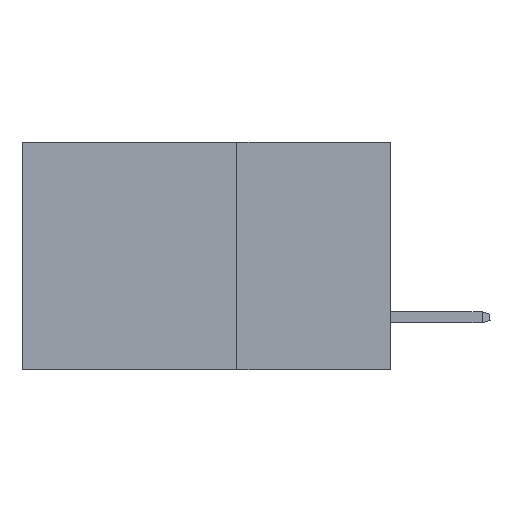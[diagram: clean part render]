
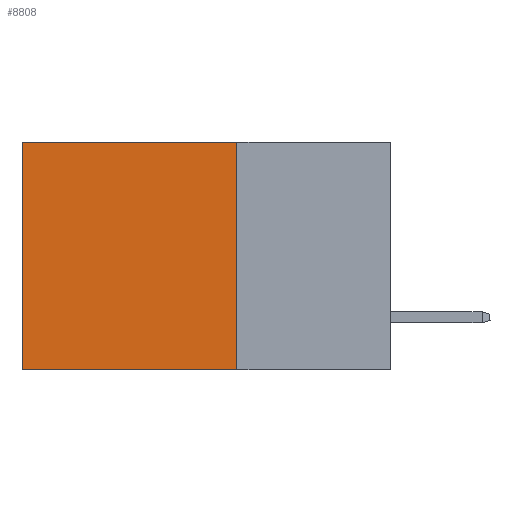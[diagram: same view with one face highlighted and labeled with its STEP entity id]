
A CAD part, left-side view. The second image highlights one B-rep face of the part: STEP entity #8808.
In plain terms, the highlighted planar face has unit normal (-1, 0, 0).
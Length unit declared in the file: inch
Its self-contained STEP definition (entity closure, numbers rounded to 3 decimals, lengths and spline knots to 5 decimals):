
#234 = EDGE_CURVE ( 'NONE', #16937, #2822, #19869, .T. ) ;
#302 = CARTESIAN_POINT ( 'NONE',  ( 0.2875, 0.6, 0. ) ) ;
#728 = CARTESIAN_POINT ( 'NONE',  ( 0.2875, 0.25, -0.37 ) ) ;
#2822 = VERTEX_POINT ( 'NONE', #15626 ) ;
#3097 = DIRECTION ( 'NONE',  ( 0., 0., -1. ) ) ;
#3258 = DIRECTION ( 'NONE',  ( 0., 0., -1. ) ) ;
#3316 = FACE_OUTER_BOUND ( 'NONE', #6712, .T. ) ;
#3740 = EDGE_CURVE ( 'NONE', #21979, #6977, #15382, .T. ) ;
#4184 = CARTESIAN_POINT ( 'NONE',  ( 0.2875, 0.25, 0. ) ) ;
#5078 = CARTESIAN_POINT ( 'NONE',  ( 0.2875, 0.6, 0. ) ) ;
#5442 = DIRECTION ( 'NONE',  ( 1., 0., 0. ) ) ;
#6490 = VECTOR ( 'NONE', #15784, 39.37008 ) ;
#6712 = EDGE_LOOP ( 'NONE', ( #21986, #18665, #23042, #12474 ) ) ;
#6977 = VERTEX_POINT ( 'NONE', #14801 ) ;
#8643 = LINE ( 'NONE', #728, #14646 ) ;
#8808 = ADVANCED_FACE ( 'NONE', ( #3316 ), #20551, .F. ) ;
#11276 = CARTESIAN_POINT ( 'NONE',  ( 0.2875, 0.25, 0. ) ) ;
#12474 = ORIENTED_EDGE ( 'NONE', *, *, #24046, .T. ) ;
#12898 = DIRECTION ( 'NONE',  ( 0., 0., -1. ) ) ;
#14646 = VECTOR ( 'NONE', #16070, 39.37008 ) ;
#14801 = CARTESIAN_POINT ( 'NONE',  ( 0.2875, 0.25, -0.37 ) ) ;
#15382 = LINE ( 'NONE', #21997, #22581 ) ;
#15522 = LINE ( 'NONE', #4184, #6490 ) ;
#15626 = CARTESIAN_POINT ( 'NONE',  ( 0.2875, 0.6, -0.37 ) ) ;
#15659 = VECTOR ( 'NONE', #3258, 39.37008 ) ;
#15784 = DIRECTION ( 'NONE',  ( 0., 1., 0. ) ) ;
#16070 = DIRECTION ( 'NONE',  ( 0., 1., 0. ) ) ;
#16937 = VERTEX_POINT ( 'NONE', #302 ) ;
#17212 = AXIS2_PLACEMENT_3D ( 'NONE', #11276, #5442, #12898 ) ;
#18665 = ORIENTED_EDGE ( 'NONE', *, *, #23436, .F. ) ;
#19869 = LINE ( 'NONE', #5078, #15659 ) ;
#20551 = PLANE ( 'NONE',  #17212 ) ;
#21979 = VERTEX_POINT ( 'NONE', #23151 ) ;
#21986 = ORIENTED_EDGE ( 'NONE', *, *, #234, .T. ) ;
#21997 = CARTESIAN_POINT ( 'NONE',  ( 0.2875, 0.25, 0. ) ) ;
#22581 = VECTOR ( 'NONE', #3097, 39.37008 ) ;
#23042 = ORIENTED_EDGE ( 'NONE', *, *, #3740, .F. ) ;
#23151 = CARTESIAN_POINT ( 'NONE',  ( 0.2875, 0.25, 0. ) ) ;
#23436 = EDGE_CURVE ( 'NONE', #6977, #2822, #8643, .T. ) ;
#24046 = EDGE_CURVE ( 'NONE', #21979, #16937, #15522, .T. ) ;
